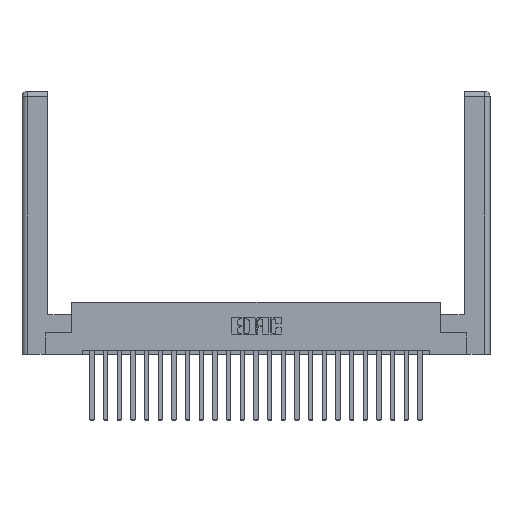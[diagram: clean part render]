
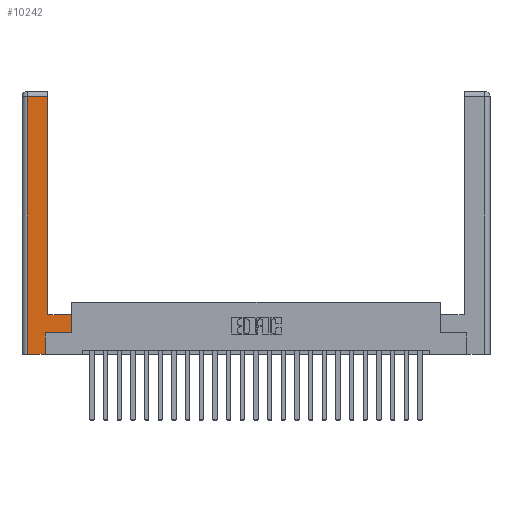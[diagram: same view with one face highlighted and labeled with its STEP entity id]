
A CAD part, top view. The second image highlights one B-rep face of the part: STEP entity #10242.
In plain terms, the highlighted planar face has unit normal (0, 0, 1).
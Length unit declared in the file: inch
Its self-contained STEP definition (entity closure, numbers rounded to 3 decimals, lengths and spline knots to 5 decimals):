
#34 = LINE ( 'NONE', #23427, #19795 ) ;
#1045 = DIRECTION ( 'NONE',  ( -1., 0., 0. ) ) ;
#1181 = VECTOR ( 'NONE', #19777, 39.37008 ) ;
#1758 = LINE ( 'NONE', #3068, #1181 ) ;
#2039 = CARTESIAN_POINT ( 'NONE',  ( 0.565, 0.245, 0. ) ) ;
#2537 = EDGE_CURVE ( 'NONE', #13529, #21236, #34, .T. ) ;
#2649 = DIRECTION ( 'NONE',  ( 0., 1., 0. ) ) ;
#2731 = ORIENTED_EDGE ( 'NONE', *, *, #2537, .T. ) ;
#3007 = LINE ( 'NONE', #2039, #22739 ) ;
#3068 = CARTESIAN_POINT ( 'NONE',  ( 0.265, 0., 0. ) ) ;
#3330 = CARTESIAN_POINT ( 'NONE',  ( 0.0615, 0., 0. ) ) ;
#3385 = CARTESIAN_POINT ( 'NONE',  ( 0.295, 0.45, 0. ) ) ;
#3640 = LINE ( 'NONE', #22095, #23418 ) ;
#3749 = EDGE_CURVE ( 'NONE', #21236, #16964, #19477, .T. ) ;
#3885 = EDGE_CURVE ( 'NONE', #16964, #10125, #1758, .T. ) ;
#4031 = CARTESIAN_POINT ( 'NONE',  ( 0.565, 0.45, 0. ) ) ;
#4459 = ORIENTED_EDGE ( 'NONE', *, *, #23825, .T. ) ;
#4528 = DIRECTION ( 'NONE',  ( -1., 0., 0. ) ) ;
#4797 = AXIS2_PLACEMENT_3D ( 'NONE', #15711, #16030, #1045 ) ;
#5544 = VERTEX_POINT ( 'NONE', #4031 ) ;
#5580 = DIRECTION ( 'NONE',  ( 0., 1., 0. ) ) ;
#5800 = VECTOR ( 'NONE', #6689, 39.37008 ) ;
#6071 = CARTESIAN_POINT ( 'NONE',  ( 0.565, 0.45, 0. ) ) ;
#6333 = EDGE_CURVE ( 'NONE', #10125, #12660, #3640, .T. ) ;
#6606 = CARTESIAN_POINT ( 'NONE',  ( 0.0615, 0., 0. ) ) ;
#6689 = DIRECTION ( 'NONE',  ( 0., -1., 0. ) ) ;
#7131 = LINE ( 'NONE', #8154, #23997 ) ;
#8119 = ORIENTED_EDGE ( 'NONE', *, *, #10164, .T. ) ;
#8154 = CARTESIAN_POINT ( 'NONE',  ( 0.295, 3., 0. ) ) ;
#8343 = EDGE_CURVE ( 'NONE', #12660, #20267, #3007, .T. ) ;
#8988 = CARTESIAN_POINT ( 'NONE',  ( 0.265, 0.245, 0. ) ) ;
#10025 = CARTESIAN_POINT ( 'NONE',  ( 0.295, 0.45, 0. ) ) ;
#10125 = VERTEX_POINT ( 'NONE', #14905 ) ;
#10164 = EDGE_CURVE ( 'NONE', #5544, #18577, #16774, .T. ) ;
#10242 = ADVANCED_FACE ( 'NONE', ( #20590 ), #11659, .F. ) ;
#10258 = ORIENTED_EDGE ( 'NONE', *, *, #6333, .T. ) ;
#11508 = DIRECTION ( 'NONE',  ( 0., 1., 0. ) ) ;
#11659 = PLANE ( 'NONE',  #4797 ) ;
#11937 = CARTESIAN_POINT ( 'NONE',  ( 0.295, 2.94, 0. ) ) ;
#12097 = EDGE_CURVE ( 'NONE', #18577, #13529, #7131, .T. ) ;
#12280 = ORIENTED_EDGE ( 'NONE', *, *, #3749, .T. ) ;
#12660 = VERTEX_POINT ( 'NONE', #8988 ) ;
#12744 = CARTESIAN_POINT ( 'NONE',  ( 0.0615, 2.94, 0. ) ) ;
#13529 = VERTEX_POINT ( 'NONE', #11937 ) ;
#14060 = VECTOR ( 'NONE', #11508, 39.37008 ) ;
#14635 = LINE ( 'NONE', #6071, #14060 ) ;
#14905 = CARTESIAN_POINT ( 'NONE',  ( 0.265, 0., 0. ) ) ;
#15078 = DIRECTION ( 'NONE',  ( 1., 0., 0. ) ) ;
#15711 = CARTESIAN_POINT ( 'NONE',  ( 0., 0., 0. ) ) ;
#15885 = ORIENTED_EDGE ( 'NONE', *, *, #3885, .T. ) ;
#16030 = DIRECTION ( 'NONE',  ( 0., 0., -1. ) ) ;
#16289 = EDGE_LOOP ( 'NONE', ( #21721, #2731, #12280, #15885, #10258, #18528, #4459, #8119 ) ) ;
#16774 = LINE ( 'NONE', #10025, #17673 ) ;
#16964 = VERTEX_POINT ( 'NONE', #3330 ) ;
#17673 = VECTOR ( 'NONE', #4528, 39.37008 ) ;
#18528 = ORIENTED_EDGE ( 'NONE', *, *, #8343, .T. ) ;
#18577 = VERTEX_POINT ( 'NONE', #3385 ) ;
#19477 = LINE ( 'NONE', #6606, #5800 ) ;
#19777 = DIRECTION ( 'NONE',  ( 1., 0., 0. ) ) ;
#19795 = VECTOR ( 'NONE', #21310, 39.37008 ) ;
#20267 = VERTEX_POINT ( 'NONE', #22089 ) ;
#20590 = FACE_OUTER_BOUND ( 'NONE', #16289, .T. ) ;
#21236 = VERTEX_POINT ( 'NONE', #12744 ) ;
#21310 = DIRECTION ( 'NONE',  ( -1., 0., 0. ) ) ;
#21721 = ORIENTED_EDGE ( 'NONE', *, *, #12097, .T. ) ;
#22089 = CARTESIAN_POINT ( 'NONE',  ( 0.565, 0.245, 0. ) ) ;
#22095 = CARTESIAN_POINT ( 'NONE',  ( 0.265, 0.245, 0. ) ) ;
#22739 = VECTOR ( 'NONE', #15078, 39.37008 ) ;
#23418 = VECTOR ( 'NONE', #5580, 39.37008 ) ;
#23427 = CARTESIAN_POINT ( 'NONE',  ( 0.0615, 2.94, 0. ) ) ;
#23825 = EDGE_CURVE ( 'NONE', #20267, #5544, #14635, .T. ) ;
#23997 = VECTOR ( 'NONE', #2649, 39.37008 ) ;
